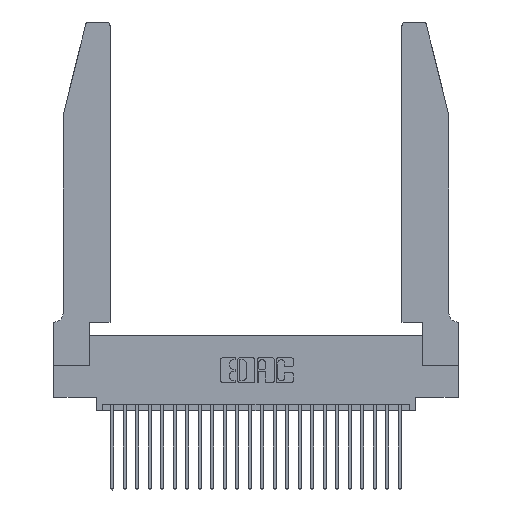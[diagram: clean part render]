
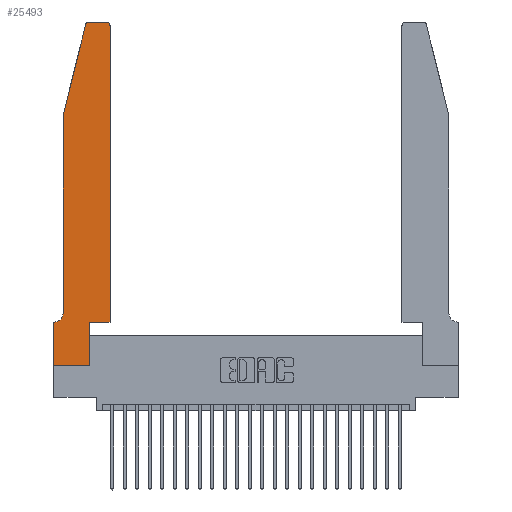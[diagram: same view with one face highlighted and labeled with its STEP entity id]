
A CAD part, top view. The second image highlights one B-rep face of the part: STEP entity #25493.
In plain terms, the highlighted planar face has unit normal (0, 0, 1).
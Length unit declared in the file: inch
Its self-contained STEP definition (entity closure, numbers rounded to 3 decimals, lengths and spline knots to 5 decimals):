
#90 = VERTEX_POINT ( 'NONE', #23461 ) ;
#259 = CARTESIAN_POINT ( 'NONE',  ( 0.0755, 0.42, 0.37 ) ) ;
#443 = CARTESIAN_POINT ( 'NONE',  ( 0.0755, 2., 0.37 ) ) ;
#793 = VERTEX_POINT ( 'NONE', #20598 ) ;
#1562 = CARTESIAN_POINT ( 'NONE',  ( 0.0055, 0.42, 0.37 ) ) ;
#1765 = VERTEX_POINT ( 'NONE', #22922 ) ;
#1769 = DIRECTION ( 'NONE',  ( 0., 1., 0. ) ) ;
#1916 = VERTEX_POINT ( 'NONE', #13068 ) ;
#2076 = EDGE_LOOP ( 'NONE', ( #6632, #2844, #12691, #23555, #4068, #6883, #19401, #16202, #13212, #5903, #14398, #19082 ) ) ;
#2121 = DIRECTION ( 'NONE',  ( 1., 0., 0. ) ) ;
#2844 = ORIENTED_EDGE ( 'NONE', *, *, #22550, .T. ) ;
#3472 = VERTEX_POINT ( 'NONE', #22689 ) ;
#4068 = ORIENTED_EDGE ( 'NONE', *, *, #13991, .T. ) ;
#4181 = DIRECTION ( 'NONE',  ( 0., -1., 0. ) ) ;
#4561 = CARTESIAN_POINT ( 'NONE',  ( 0.4205, 2.75, 0.37 ) ) ;
#4650 = LINE ( 'NONE', #22028, #13157 ) ;
#4914 = DIRECTION ( 'NONE',  ( -1., 0., 0. ) ) ;
#5066 = CARTESIAN_POINT ( 'NONE',  ( 0.4505, 0.35, 0.37 ) ) ;
#5109 = VERTEX_POINT ( 'NONE', #21347 ) ;
#5224 = DIRECTION ( 'NONE',  ( 0., 0., 1. ) ) ;
#5903 = ORIENTED_EDGE ( 'NONE', *, *, #9317, .T. ) ;
#5998 = VERTEX_POINT ( 'NONE', #259 ) ;
#6238 = EDGE_CURVE ( 'NONE', #3472, #90, #4650, .T. ) ;
#6448 = VECTOR ( 'NONE', #1769, 39.37008 ) ;
#6552 = LINE ( 'NONE', #15929, #24224 ) ;
#6632 = ORIENTED_EDGE ( 'NONE', *, *, #16683, .T. ) ;
#6883 = ORIENTED_EDGE ( 'NONE', *, *, #12528, .T. ) ;
#7156 = DIRECTION ( 'NONE',  ( 1., 0., 0. ) ) ;
#7410 = CIRCLE ( 'NONE', #10741, 0.03 ) ;
#7690 = VECTOR ( 'NONE', #23264, 39.37008 ) ;
#8118 = CARTESIAN_POINT ( 'NONE',  ( 0.0755, 2., 0.37 ) ) ;
#8333 = DIRECTION ( 'NONE',  ( 1., 0., 0. ) ) ;
#8467 = EDGE_CURVE ( 'NONE', #1765, #16671, #16095, .T. ) ;
#8597 = DIRECTION ( 'NONE',  ( 0., 0., 1. ) ) ;
#8736 = VECTOR ( 'NONE', #14257, 39.37008 ) ;
#8885 = CARTESIAN_POINT ( 'NONE',  ( 0.284, 2.72, 0.37 ) ) ;
#9317 = EDGE_CURVE ( 'NONE', #16025, #18765, #10060, .T. ) ;
#10060 = LINE ( 'NONE', #24500, #19856 ) ;
#10598 = DIRECTION ( 'NONE',  ( 1., 0., 0. ) ) ;
#10741 = AXIS2_PLACEMENT_3D ( 'NONE', #8885, #23037, #21266 ) ;
#10863 = VECTOR ( 'NONE', #10958, 39.37008 ) ;
#10915 = CARTESIAN_POINT ( 'NONE',  ( 0.2865, 0.35, 0.37 ) ) ;
#10958 = DIRECTION ( 'NONE',  ( -1., 0., 0. ) ) ;
#11082 = LINE ( 'NONE', #25028, #12347 ) ;
#11240 = VERTEX_POINT ( 'NONE', #16296 ) ;
#11651 = DIRECTION ( 'NONE',  ( 0., 0., -1. ) ) ;
#12347 = VECTOR ( 'NONE', #4914, 39.37008 ) ;
#12528 = EDGE_CURVE ( 'NONE', #5109, #3472, #22582, .T. ) ;
#12691 = ORIENTED_EDGE ( 'NONE', *, *, #19802, .T. ) ;
#13068 = CARTESIAN_POINT ( 'NONE',  ( 0.0755, 2., 0.37 ) ) ;
#13157 = VECTOR ( 'NONE', #4181, 39.37008 ) ;
#13212 = ORIENTED_EDGE ( 'NONE', *, *, #15182, .T. ) ;
#13477 = CARTESIAN_POINT ( 'NONE',  ( 0.284, 2.75, 0.37 ) ) ;
#13991 = EDGE_CURVE ( 'NONE', #5998, #5109, #18711, .T. ) ;
#14257 = DIRECTION ( 'NONE',  ( -0.239, -0.971, 0. ) ) ;
#14398 = ORIENTED_EDGE ( 'NONE', *, *, #23329, .T. ) ;
#14963 = EDGE_CURVE ( 'NONE', #90, #11240, #6552, .T. ) ;
#15182 = EDGE_CURVE ( 'NONE', #11240, #16025, #24742, .T. ) ;
#15929 = CARTESIAN_POINT ( 'NONE',  ( 0., 0., 0.37 ) ) ;
#16025 = VERTEX_POINT ( 'NONE', #10915 ) ;
#16095 = CIRCLE ( 'NONE', #18573, 0.03 ) ;
#16202 = ORIENTED_EDGE ( 'NONE', *, *, #14963, .T. ) ;
#16296 = CARTESIAN_POINT ( 'NONE',  ( 0.2865, 0., 0.37 ) ) ;
#16354 = DIRECTION ( 'NONE',  ( 0., -1., 0. ) ) ;
#16671 = VERTEX_POINT ( 'NONE', #4561 ) ;
#16683 = EDGE_CURVE ( 'NONE', #16671, #22102, #11082, .T. ) ;
#17283 = LINE ( 'NONE', #443, #8736 ) ;
#17496 = PLANE ( 'NONE',  #24692 ) ;
#17903 = CARTESIAN_POINT ( 'NONE',  ( 0.2865, 0.35, 0.37 ) ) ;
#18144 = AXIS2_PLACEMENT_3D ( 'NONE', #1562, #11651, #23896 ) ;
#18151 = VECTOR ( 'NONE', #16354, 39.37008 ) ;
#18573 = AXIS2_PLACEMENT_3D ( 'NONE', #20745, #8597, #10598 ) ;
#18711 = CIRCLE ( 'NONE', #18144, 0.07 ) ;
#18765 = VERTEX_POINT ( 'NONE', #18932 ) ;
#18932 = CARTESIAN_POINT ( 'NONE',  ( 0.4505, 0.35, 0.37 ) ) ;
#19082 = ORIENTED_EDGE ( 'NONE', *, *, #8467, .T. ) ;
#19401 = ORIENTED_EDGE ( 'NONE', *, *, #6238, .T. ) ;
#19802 = EDGE_CURVE ( 'NONE', #793, #1916, #17283, .T. ) ;
#19856 = VECTOR ( 'NONE', #8333, 39.37008 ) ;
#20598 = CARTESIAN_POINT ( 'NONE',  ( 0.25487, 2.72718, 0.37 ) ) ;
#20745 = CARTESIAN_POINT ( 'NONE',  ( 0.4205, 2.72, 0.37 ) ) ;
#21266 = DIRECTION ( 'NONE',  ( 1., 0., 0. ) ) ;
#21297 = CARTESIAN_POINT ( 'NONE',  ( 0., 0.35, 0.37 ) ) ;
#21347 = CARTESIAN_POINT ( 'NONE',  ( 0.0055, 0.35, 0.37 ) ) ;
#21684 = EDGE_CURVE ( 'NONE', #1916, #5998, #25333, .T. ) ;
#22028 = CARTESIAN_POINT ( 'NONE',  ( 0., 0., 0.37 ) ) ;
#22102 = VERTEX_POINT ( 'NONE', #13477 ) ;
#22217 = CARTESIAN_POINT ( 'NONE',  ( 0.0755, 0.35, 0.37 ) ) ;
#22450 = FACE_OUTER_BOUND ( 'NONE', #2076, .T. ) ;
#22550 = EDGE_CURVE ( 'NONE', #22102, #793, #7410, .T. ) ;
#22582 = LINE ( 'NONE', #22217, #10863 ) ;
#22689 = CARTESIAN_POINT ( 'NONE',  ( 0., 0.35, 0.37 ) ) ;
#22922 = CARTESIAN_POINT ( 'NONE',  ( 0.4505, 2.72, 0.37 ) ) ;
#23037 = DIRECTION ( 'NONE',  ( 0., 0., 1. ) ) ;
#23264 = DIRECTION ( 'NONE',  ( 0., 1., 0. ) ) ;
#23329 = EDGE_CURVE ( 'NONE', #18765, #1765, #24762, .T. ) ;
#23461 = CARTESIAN_POINT ( 'NONE',  ( 0., 0., 0.37 ) ) ;
#23555 = ORIENTED_EDGE ( 'NONE', *, *, #21684, .T. ) ;
#23896 = DIRECTION ( 'NONE',  ( -1., 0., 0. ) ) ;
#24224 = VECTOR ( 'NONE', #2121, 39.37008 ) ;
#24500 = CARTESIAN_POINT ( 'NONE',  ( 0.4505, 0.35, 0.37 ) ) ;
#24692 = AXIS2_PLACEMENT_3D ( 'NONE', #21297, #5224, #7156 ) ;
#24742 = LINE ( 'NONE', #17903, #6448 ) ;
#24762 = LINE ( 'NONE', #5066, #7690 ) ;
#25028 = CARTESIAN_POINT ( 'NONE',  ( 0.2605, 2.75, 0.37 ) ) ;
#25333 = LINE ( 'NONE', #8118, #18151 ) ;
#25493 = ADVANCED_FACE ( 'NONE', ( #22450 ), #17496, .T. ) ;
